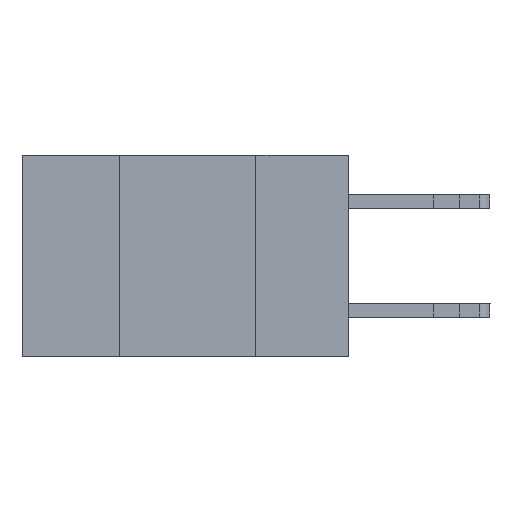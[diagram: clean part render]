
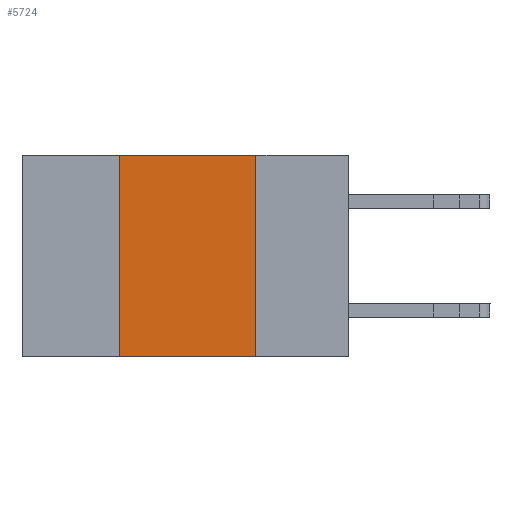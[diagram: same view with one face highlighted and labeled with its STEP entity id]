
A CAD part, left-side view. The second image highlights one B-rep face of the part: STEP entity #5724.
In plain terms, the highlighted planar face has unit normal (-1, 0, 0).
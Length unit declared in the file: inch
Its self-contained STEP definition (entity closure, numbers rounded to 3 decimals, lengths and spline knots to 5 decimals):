
#71 = CARTESIAN_POINT ( 'NONE',  ( 0., 0.6, -0.37 ) ) ;
#147 = VECTOR ( 'NONE', #21104, 39.37008 ) ;
#757 = DIRECTION ( 'NONE',  ( 0., 0., -1. ) ) ;
#1136 = DIRECTION ( 'NONE',  ( 0., -1., 0. ) ) ;
#1504 = LINE ( 'NONE', #13506, #13450 ) ;
#3771 = CARTESIAN_POINT ( 'NONE',  ( 0., 0.17, 0. ) ) ;
#4165 = CARTESIAN_POINT ( 'NONE',  ( 0., 0.17, -0.37 ) ) ;
#4264 = ORIENTED_EDGE ( 'NONE', *, *, #24235, .F. ) ;
#5595 = LINE ( 'NONE', #21273, #147 ) ;
#5724 = ADVANCED_FACE ( 'NONE', ( #8445 ), #6877, .F. ) ;
#6877 = PLANE ( 'NONE',  #22390 ) ;
#7700 = CARTESIAN_POINT ( 'NONE',  ( 0., 0.42, 0. ) ) ;
#8445 = FACE_OUTER_BOUND ( 'NONE', #24149, .T. ) ;
#8664 = VERTEX_POINT ( 'NONE', #11051 ) ;
#9182 = VERTEX_POINT ( 'NONE', #10290 ) ;
#9319 = VECTOR ( 'NONE', #14392, 39.37008 ) ;
#10290 = CARTESIAN_POINT ( 'NONE',  ( 0., 0.42, -0.37 ) ) ;
#10326 = DIRECTION ( 'NONE',  ( 0., 0., 1. ) ) ;
#10511 = VECTOR ( 'NONE', #10326, 39.37008 ) ;
#10854 = CARTESIAN_POINT ( 'NONE',  ( 0., 0.6, 0. ) ) ;
#10949 = EDGE_CURVE ( 'NONE', #18828, #17762, #5595, .T. ) ;
#11051 = CARTESIAN_POINT ( 'NONE',  ( 0., 0.42, 0. ) ) ;
#11890 = LINE ( 'NONE', #71, #9319 ) ;
#13450 = VECTOR ( 'NONE', #1136, 39.37008 ) ;
#13506 = CARTESIAN_POINT ( 'NONE',  ( 0., 0.6, 0. ) ) ;
#13887 = ORIENTED_EDGE ( 'NONE', *, *, #10949, .F. ) ;
#14392 = DIRECTION ( 'NONE',  ( 0., -1., 0. ) ) ;
#17615 = EDGE_CURVE ( 'NONE', #9182, #8664, #20857, .T. ) ;
#17638 = ORIENTED_EDGE ( 'NONE', *, *, #17615, .F. ) ;
#17762 = VERTEX_POINT ( 'NONE', #4165 ) ;
#18362 = ORIENTED_EDGE ( 'NONE', *, *, #23147, .T. ) ;
#18828 = VERTEX_POINT ( 'NONE', #3771 ) ;
#20857 = LINE ( 'NONE', #7700, #10511 ) ;
#21104 = DIRECTION ( 'NONE',  ( 0., 0., -1. ) ) ;
#21273 = CARTESIAN_POINT ( 'NONE',  ( 0., 0.17, 0. ) ) ;
#21323 = DIRECTION ( 'NONE',  ( 1., 0., 0. ) ) ;
#22390 = AXIS2_PLACEMENT_3D ( 'NONE', #10854, #21323, #757 ) ;
#23147 = EDGE_CURVE ( 'NONE', #9182, #17762, #11890, .T. ) ;
#24149 = EDGE_LOOP ( 'NONE', ( #13887, #4264, #17638, #18362 ) ) ;
#24235 = EDGE_CURVE ( 'NONE', #8664, #18828, #1504, .T. ) ;
